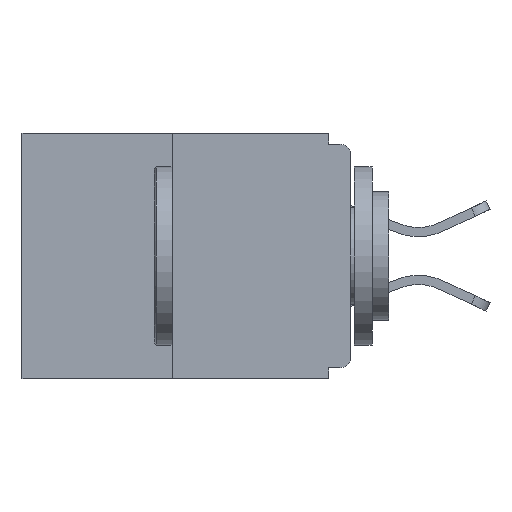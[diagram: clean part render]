
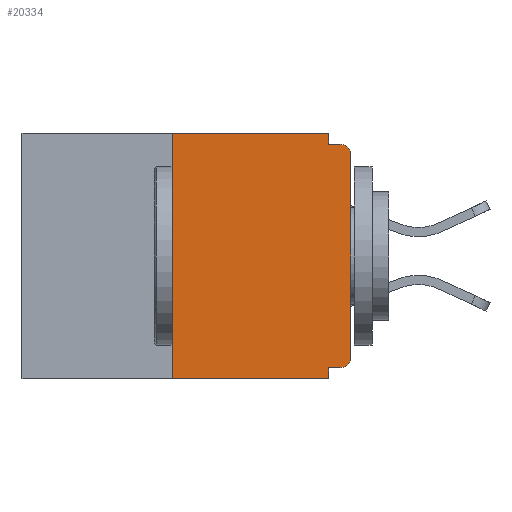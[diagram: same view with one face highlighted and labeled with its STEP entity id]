
A CAD part, left-side view. The second image highlights one B-rep face of the part: STEP entity #20334.
In plain terms, the highlighted planar face has unit normal (-1, 0, 0).
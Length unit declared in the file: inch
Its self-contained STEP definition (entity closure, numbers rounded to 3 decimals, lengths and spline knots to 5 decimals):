
#12 = AXIS2_PLACEMENT_3D ( 'NONE', #10404, #4327, #18649 ) ;
#31 = DIRECTION ( 'NONE',  ( 0., 0., 1. ) ) ;
#1057 = DIRECTION ( 'NONE',  ( 0., 0., 1. ) ) ;
#1124 = CARTESIAN_POINT ( 'NONE',  ( 0., 0.46, -0.343 ) ) ;
#1175 = CARTESIAN_POINT ( 'NONE',  ( 0., 0.031, -0.343 ) ) ;
#1240 = EDGE_CURVE ( 'NONE', #26217, #2527, #16109, .T. ) ;
#1326 = CARTESIAN_POINT ( 'NONE',  ( 0., 0.031, -0.328 ) ) ;
#1344 = CARTESIAN_POINT ( 'NONE',  ( 0., 0., -0.313 ) ) ;
#1598 = EDGE_CURVE ( 'NONE', #5364, #1950, #7437, .T. ) ;
#1950 = VERTEX_POINT ( 'NONE', #10593 ) ;
#2010 = DIRECTION ( 'NONE',  ( 1., 0., 0. ) ) ;
#2339 = LINE ( 'NONE', #21666, #2942 ) ;
#2527 = VERTEX_POINT ( 'NONE', #8214 ) ;
#2942 = VECTOR ( 'NONE', #18007, 39.37008 ) ;
#3146 = CARTESIAN_POINT ( 'NONE',  ( 0., 0., -0.328 ) ) ;
#3381 = CARTESIAN_POINT ( 'NONE',  ( 0., 0.015, -0.328 ) ) ;
#3425 = EDGE_CURVE ( 'NONE', #19315, #15696, #18302, .T. ) ;
#4132 = DIRECTION ( 'NONE',  ( 0., 0., -1. ) ) ;
#4139 = ORIENTED_EDGE ( 'NONE', *, *, #17940, .F. ) ;
#4167 = EDGE_CURVE ( 'NONE', #18741, #6853, #25657, .T. ) ;
#4327 = DIRECTION ( 'NONE',  ( -1., 0., 0. ) ) ;
#5364 = VERTEX_POINT ( 'NONE', #15646 ) ;
#5650 = CARTESIAN_POINT ( 'NONE',  ( 0., 0.031, 0. ) ) ;
#5663 = LINE ( 'NONE', #3146, #12399 ) ;
#6853 = VERTEX_POINT ( 'NONE', #1344 ) ;
#6869 = VECTOR ( 'NONE', #23373, 39.37008 ) ;
#7291 = ORIENTED_EDGE ( 'NONE', *, *, #4167, .T. ) ;
#7345 = ORIENTED_EDGE ( 'NONE', *, *, #21633, .F. ) ;
#7437 = LINE ( 'NONE', #5650, #9676 ) ;
#7594 = LINE ( 'NONE', #24660, #21988 ) ;
#7745 = VECTOR ( 'NONE', #11807, 39.37008 ) ;
#8214 = CARTESIAN_POINT ( 'NONE',  ( 0., 0.015, -0.015 ) ) ;
#9152 = EDGE_LOOP ( 'NONE', ( #4139, #7345, #20673, #12594, #20623, #7291, #25871, #14055, #14088, #19943 ) ) ;
#9251 = CARTESIAN_POINT ( 'NONE',  ( 0., 0., -0.03 ) ) ;
#9414 = EDGE_CURVE ( 'NONE', #20818, #15696, #13209, .T. ) ;
#9599 = VECTOR ( 'NONE', #23708, 39.37008 ) ;
#9676 = VECTOR ( 'NONE', #19623, 39.37008 ) ;
#10402 = EDGE_CURVE ( 'NONE', #1950, #2527, #2339, .T. ) ;
#10404 = CARTESIAN_POINT ( 'NONE',  ( 0., 0.015, -0.313 ) ) ;
#10593 = CARTESIAN_POINT ( 'NONE',  ( 0., 0.031, -0.015 ) ) ;
#11807 = DIRECTION ( 'NONE',  ( 0., -1., 0. ) ) ;
#12108 = CARTESIAN_POINT ( 'NONE',  ( 0., 0.031, -0.343 ) ) ;
#12399 = VECTOR ( 'NONE', #19590, 39.37008 ) ;
#12594 = ORIENTED_EDGE ( 'NONE', *, *, #3425, .F. ) ;
#13209 = LINE ( 'NONE', #1124, #7745 ) ;
#14021 = DIRECTION ( 'NONE',  ( 0., 0., -1. ) ) ;
#14055 = ORIENTED_EDGE ( 'NONE', *, *, #1240, .T. ) ;
#14088 = ORIENTED_EDGE ( 'NONE', *, *, #10402, .F. ) ;
#14237 = CARTESIAN_POINT ( 'NONE',  ( 0., 0.46, 0. ) ) ;
#15646 = CARTESIAN_POINT ( 'NONE',  ( 0., 0.031, 0. ) ) ;
#15696 = VERTEX_POINT ( 'NONE', #12108 ) ;
#15803 = CARTESIAN_POINT ( 'NONE',  ( 0., 0.015, -0.03 ) ) ;
#16109 = CIRCLE ( 'NONE', #18308, 0.015 ) ;
#16132 = EDGE_CURVE ( 'NONE', #6853, #26217, #7594, .T. ) ;
#16450 = CARTESIAN_POINT ( 'NONE',  ( 0., 0.25, 0. ) ) ;
#16794 = EDGE_CURVE ( 'NONE', #18741, #19315, #5663, .T. ) ;
#17667 = CARTESIAN_POINT ( 'NONE',  ( 0., 0.25, 0. ) ) ;
#17835 = CARTESIAN_POINT ( 'NONE',  ( 0., 0.25, -0.343 ) ) ;
#17940 = EDGE_CURVE ( 'NONE', #21781, #5364, #21908, .T. ) ;
#18007 = DIRECTION ( 'NONE',  ( 0., -1., 0. ) ) ;
#18302 = LINE ( 'NONE', #1175, #9599 ) ;
#18308 = AXIS2_PLACEMENT_3D ( 'NONE', #15803, #22072, #14021 ) ;
#18649 = DIRECTION ( 'NONE',  ( 0., 0., -1. ) ) ;
#18741 = VERTEX_POINT ( 'NONE', #3381 ) ;
#19315 = VERTEX_POINT ( 'NONE', #1326 ) ;
#19590 = DIRECTION ( 'NONE',  ( 0., 1., 0. ) ) ;
#19623 = DIRECTION ( 'NONE',  ( 0., 0., -1. ) ) ;
#19943 = ORIENTED_EDGE ( 'NONE', *, *, #1598, .F. ) ;
#20334 = ADVANCED_FACE ( 'NONE', ( #23535 ), #24654, .F. ) ;
#20623 = ORIENTED_EDGE ( 'NONE', *, *, #16794, .F. ) ;
#20673 = ORIENTED_EDGE ( 'NONE', *, *, #9414, .T. ) ;
#20818 = VERTEX_POINT ( 'NONE', #17835 ) ;
#21633 = EDGE_CURVE ( 'NONE', #20818, #21781, #25074, .T. ) ;
#21666 = CARTESIAN_POINT ( 'NONE',  ( 0., 0., -0.015 ) ) ;
#21781 = VERTEX_POINT ( 'NONE', #16450 ) ;
#21908 = LINE ( 'NONE', #23198, #6869 ) ;
#21988 = VECTOR ( 'NONE', #31, 39.37008 ) ;
#22072 = DIRECTION ( 'NONE',  ( -1., 0., 0. ) ) ;
#23198 = CARTESIAN_POINT ( 'NONE',  ( 0., 0.46, 0. ) ) ;
#23373 = DIRECTION ( 'NONE',  ( 0., -1., 0. ) ) ;
#23535 = FACE_OUTER_BOUND ( 'NONE', #9152, .T. ) ;
#23708 = DIRECTION ( 'NONE',  ( 0., 0., -1. ) ) ;
#23739 = AXIS2_PLACEMENT_3D ( 'NONE', #14237, #2010, #4132 ) ;
#24426 = VECTOR ( 'NONE', #1057, 39.37008 ) ;
#24654 = PLANE ( 'NONE',  #23739 ) ;
#24660 = CARTESIAN_POINT ( 'NONE',  ( 0., 0., 0. ) ) ;
#25074 = LINE ( 'NONE', #17667, #24426 ) ;
#25657 = CIRCLE ( 'NONE', #12, 0.015 ) ;
#25871 = ORIENTED_EDGE ( 'NONE', *, *, #16132, .T. ) ;
#26217 = VERTEX_POINT ( 'NONE', #9251 ) ;
